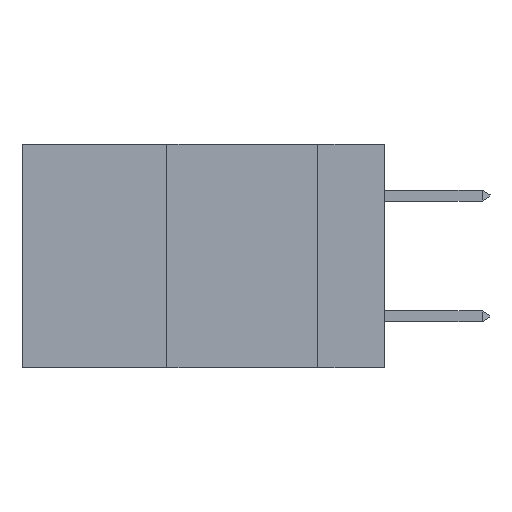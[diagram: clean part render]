
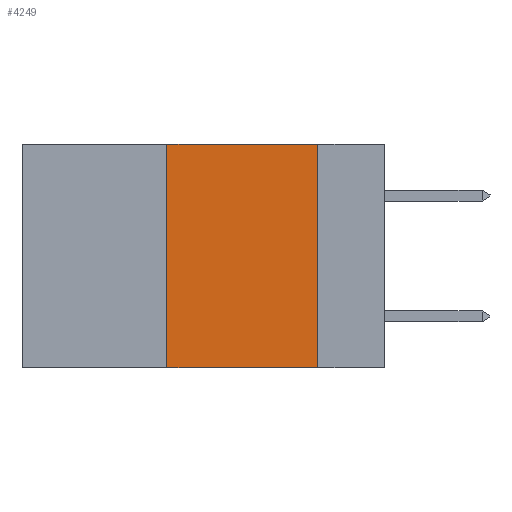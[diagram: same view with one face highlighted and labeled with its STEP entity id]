
A CAD part, left-side view. The second image highlights one B-rep face of the part: STEP entity #4249.
In plain terms, the highlighted planar face has unit normal (-1, 0, 0).
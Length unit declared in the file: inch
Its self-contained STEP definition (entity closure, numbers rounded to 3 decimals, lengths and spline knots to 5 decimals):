
#10 = EDGE_CURVE ( 'NONE', #10984, #11154, #11218, .T. ) ;
#42 = CARTESIAN_POINT ( 'NONE',  ( 0., 0.6, 0. ) ) ;
#621 = CARTESIAN_POINT ( 'NONE',  ( 0., 0.6, -0.37 ) ) ;
#672 = DIRECTION ( 'NONE',  ( 0., 0., -1. ) ) ;
#910 = CARTESIAN_POINT ( 'NONE',  ( 0., 0.11, 0. ) ) ;
#1032 = DIRECTION ( 'NONE',  ( 1., 0., 0. ) ) ;
#2049 = CARTESIAN_POINT ( 'NONE',  ( 0., 0.11, -0.37 ) ) ;
#2259 = FACE_OUTER_BOUND ( 'NONE', #6608, .T. ) ;
#3320 = DIRECTION ( 'NONE',  ( 0., -1., 0. ) ) ;
#4034 = LINE ( 'NONE', #8209, #6190 ) ;
#4249 = ADVANCED_FACE ( 'NONE', ( #2259 ), #11717, .F. ) ;
#4306 = LINE ( 'NONE', #621, #6466 ) ;
#4379 = ORIENTED_EDGE ( 'NONE', *, *, #10, .F. ) ;
#4506 = CARTESIAN_POINT ( 'NONE',  ( 0., 0.11, 0. ) ) ;
#4772 = ORIENTED_EDGE ( 'NONE', *, *, #9952, .F. ) ;
#5423 = VERTEX_POINT ( 'NONE', #2049 ) ;
#5690 = ORIENTED_EDGE ( 'NONE', *, *, #9898, .T. ) ;
#6190 = VECTOR ( 'NONE', #9142, 39.37008 ) ;
#6466 = VECTOR ( 'NONE', #8155, 39.37008 ) ;
#6608 = EDGE_LOOP ( 'NONE', ( #4772, #4379, #10922, #5690 ) ) ;
#6748 = LINE ( 'NONE', #4506, #8334 ) ;
#7494 = CARTESIAN_POINT ( 'NONE',  ( 0., 0.36, -0.37 ) ) ;
#7549 = DIRECTION ( 'NONE',  ( 0., 0., -1. ) ) ;
#8155 = DIRECTION ( 'NONE',  ( 0., -1., 0. ) ) ;
#8209 = CARTESIAN_POINT ( 'NONE',  ( 0., 0.36, 0. ) ) ;
#8334 = VECTOR ( 'NONE', #672, 39.37008 ) ;
#8418 = VERTEX_POINT ( 'NONE', #7494 ) ;
#8474 = CARTESIAN_POINT ( 'NONE',  ( 0., 0.6, 0. ) ) ;
#8985 = CARTESIAN_POINT ( 'NONE',  ( 0., 0.36, 0. ) ) ;
#9008 = AXIS2_PLACEMENT_3D ( 'NONE', #8474, #1032, #7549 ) ;
#9119 = VECTOR ( 'NONE', #3320, 39.37008 ) ;
#9142 = DIRECTION ( 'NONE',  ( 0., 0., 1. ) ) ;
#9898 = EDGE_CURVE ( 'NONE', #8418, #5423, #4306, .T. ) ;
#9932 = EDGE_CURVE ( 'NONE', #8418, #10984, #4034, .T. ) ;
#9952 = EDGE_CURVE ( 'NONE', #11154, #5423, #6748, .T. ) ;
#10922 = ORIENTED_EDGE ( 'NONE', *, *, #9932, .F. ) ;
#10984 = VERTEX_POINT ( 'NONE', #8985 ) ;
#11154 = VERTEX_POINT ( 'NONE', #910 ) ;
#11218 = LINE ( 'NONE', #42, #9119 ) ;
#11717 = PLANE ( 'NONE',  #9008 ) ;
